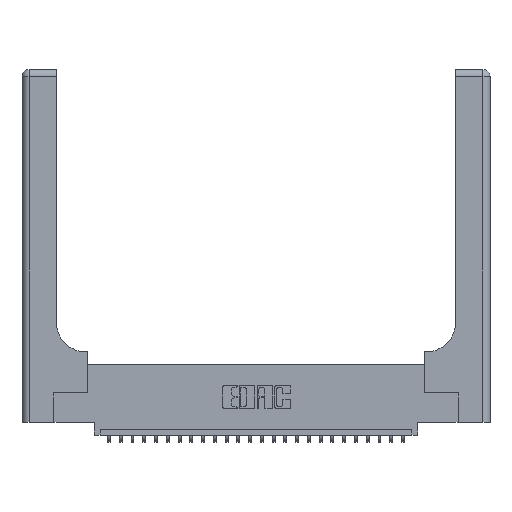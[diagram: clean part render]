
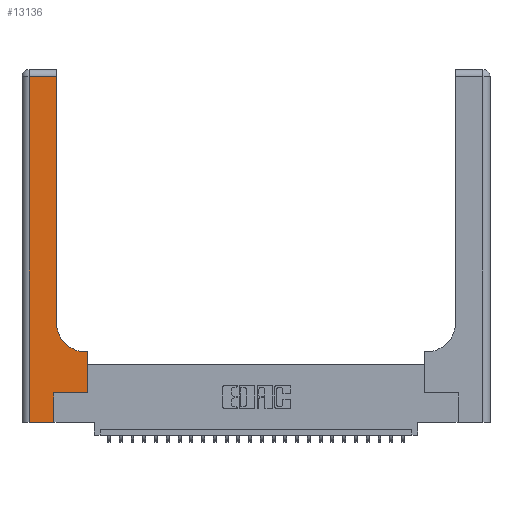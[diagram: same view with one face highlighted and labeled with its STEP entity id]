
A CAD part, top view. The second image highlights one B-rep face of the part: STEP entity #13136.
In plain terms, the highlighted planar face has unit normal (0, 0, 1).
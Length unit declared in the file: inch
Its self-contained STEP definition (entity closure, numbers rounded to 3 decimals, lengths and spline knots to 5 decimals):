
#237 = CARTESIAN_POINT ( 'NONE',  ( 0.5415, 0.85, 0.37 ) ) ;
#537 = LINE ( 'NONE', #4681, #21188 ) ;
#822 = DIRECTION ( 'NONE',  ( 1., 0., 0. ) ) ;
#1306 = DIRECTION ( 'NONE',  ( 0., 0., -1. ) ) ;
#1953 = VECTOR ( 'NONE', #10966, 39.37008 ) ;
#1999 = CARTESIAN_POINT ( 'NONE',  ( 0.5415, 0.6, 0.37 ) ) ;
#2182 = ORIENTED_EDGE ( 'NONE', *, *, #2912, .T. ) ;
#2410 = AXIS2_PLACEMENT_3D ( 'NONE', #5338, #1306, #20167 ) ;
#2506 = EDGE_CURVE ( 'NONE', #6646, #26910, #22840, .T. ) ;
#2912 = EDGE_CURVE ( 'NONE', #25983, #12294, #5757, .T. ) ;
#3246 = LINE ( 'NONE', #12802, #1953 ) ;
#3603 = ORIENTED_EDGE ( 'NONE', *, *, #12287, .T. ) ;
#3618 = CARTESIAN_POINT ( 'NONE',  ( 0.2915, 2.94, 0.37 ) ) ;
#3941 = DIRECTION ( 'NONE',  ( -1., 0., 0. ) ) ;
#4486 = DIRECTION ( 'NONE',  ( 0., 1., 0. ) ) ;
#4508 = LINE ( 'NONE', #7387, #11407 ) ;
#4681 = CARTESIAN_POINT ( 'NONE',  ( 0.5585, 0.25, 0.37 ) ) ;
#4763 = CARTESIAN_POINT ( 'NONE',  ( 0.2915, 3., 0.37 ) ) ;
#4790 = CARTESIAN_POINT ( 'NONE',  ( 0.06, 2.94, 0.37 ) ) ;
#5338 = CARTESIAN_POINT ( 'NONE',  ( 0., 3., 0.37 ) ) ;
#5757 = LINE ( 'NONE', #4763, #17895 ) ;
#5936 = VERTEX_POINT ( 'NONE', #4790 ) ;
#6084 = ORIENTED_EDGE ( 'NONE', *, *, #8447, .T. ) ;
#6435 = AXIS2_PLACEMENT_3D ( 'NONE', #237, #8864, #14892 ) ;
#6646 = VERTEX_POINT ( 'NONE', #12034 ) ;
#7387 = CARTESIAN_POINT ( 'NONE',  ( 0., 0., 0.37 ) ) ;
#8447 = EDGE_CURVE ( 'NONE', #12294, #5936, #3246, .T. ) ;
#8834 = LINE ( 'NONE', #15126, #18684 ) ;
#8864 = DIRECTION ( 'NONE',  ( 0., 0., -1. ) ) ;
#9671 = LINE ( 'NONE', #18732, #20826 ) ;
#9873 = EDGE_CURVE ( 'NONE', #15665, #22065, #4508, .T. ) ;
#10474 = ORIENTED_EDGE ( 'NONE', *, *, #18932, .T. ) ;
#10754 = ORIENTED_EDGE ( 'NONE', *, *, #13555, .T. ) ;
#10966 = DIRECTION ( 'NONE',  ( -1., 0., 0. ) ) ;
#11407 = VECTOR ( 'NONE', #822, 39.37008 ) ;
#12034 = CARTESIAN_POINT ( 'NONE',  ( 0.5585, 0.6, 0.37 ) ) ;
#12086 = ORIENTED_EDGE ( 'NONE', *, *, #2506, .T. ) ;
#12287 = EDGE_CURVE ( 'NONE', #5936, #15665, #21203, .T. ) ;
#12294 = VERTEX_POINT ( 'NONE', #3618 ) ;
#12598 = ORIENTED_EDGE ( 'NONE', *, *, #12621, .T. ) ;
#12621 = EDGE_CURVE ( 'NONE', #26910, #25983, #21809, .T. ) ;
#12698 = VECTOR ( 'NONE', #3941, 39.37008 ) ;
#12802 = CARTESIAN_POINT ( 'NONE',  ( 0., 2.94, 0.37 ) ) ;
#13095 = DIRECTION ( 'NONE',  ( 0., 1., 0. ) ) ;
#13136 = ADVANCED_FACE ( 'NONE', ( #26436 ), #19986, .F. ) ;
#13555 = EDGE_CURVE ( 'NONE', #19048, #6646, #537, .T. ) ;
#14058 = CARTESIAN_POINT ( 'NONE',  ( 0.06, 0., 0.37 ) ) ;
#14331 = CARTESIAN_POINT ( 'NONE',  ( 0.269, 0.25, 0.37 ) ) ;
#14892 = DIRECTION ( 'NONE',  ( 1., 0., 0. ) ) ;
#15126 = CARTESIAN_POINT ( 'NONE',  ( 0.269, 0.25, 0.37 ) ) ;
#15665 = VERTEX_POINT ( 'NONE', #14058 ) ;
#16146 = EDGE_LOOP ( 'NONE', ( #2182, #6084, #3603, #19622, #25706, #10474, #10754, #12086, #12598 ) ) ;
#16540 = CARTESIAN_POINT ( 'NONE',  ( 0.269, 0., 0.37 ) ) ;
#17895 = VECTOR ( 'NONE', #4486, 39.37008 ) ;
#18531 = CARTESIAN_POINT ( 'NONE',  ( 0.2915, 0.6, 0.37 ) ) ;
#18546 = CARTESIAN_POINT ( 'NONE',  ( 0.2915, 0.85, 0.37 ) ) ;
#18684 = VECTOR ( 'NONE', #23537, 39.37008 ) ;
#18732 = CARTESIAN_POINT ( 'NONE',  ( 0.269, 0., 0.37 ) ) ;
#18932 = EDGE_CURVE ( 'NONE', #22109, #19048, #8834, .T. ) ;
#19048 = VERTEX_POINT ( 'NONE', #23894 ) ;
#19622 = ORIENTED_EDGE ( 'NONE', *, *, #9873, .T. ) ;
#19986 = PLANE ( 'NONE',  #2410 ) ;
#20167 = DIRECTION ( 'NONE',  ( -1., 0., 0. ) ) ;
#20826 = VECTOR ( 'NONE', #13095, 39.37008 ) ;
#21188 = VECTOR ( 'NONE', #24064, 39.37008 ) ;
#21203 = LINE ( 'NONE', #22013, #24433 ) ;
#21809 = CIRCLE ( 'NONE', #6435, 0.25 ) ;
#22013 = CARTESIAN_POINT ( 'NONE',  ( 0.06, 3., 0.37 ) ) ;
#22065 = VERTEX_POINT ( 'NONE', #16540 ) ;
#22109 = VERTEX_POINT ( 'NONE', #14331 ) ;
#22840 = LINE ( 'NONE', #18531, #12698 ) ;
#23537 = DIRECTION ( 'NONE',  ( 1., 0., 0. ) ) ;
#23894 = CARTESIAN_POINT ( 'NONE',  ( 0.5585, 0.25, 0.37 ) ) ;
#24064 = DIRECTION ( 'NONE',  ( 0., 1., 0. ) ) ;
#24374 = DIRECTION ( 'NONE',  ( 0., -1., 0. ) ) ;
#24433 = VECTOR ( 'NONE', #24374, 39.37008 ) ;
#25158 = EDGE_CURVE ( 'NONE', #22065, #22109, #9671, .T. ) ;
#25706 = ORIENTED_EDGE ( 'NONE', *, *, #25158, .T. ) ;
#25983 = VERTEX_POINT ( 'NONE', #18546 ) ;
#26436 = FACE_OUTER_BOUND ( 'NONE', #16146, .T. ) ;
#26910 = VERTEX_POINT ( 'NONE', #1999 ) ;
